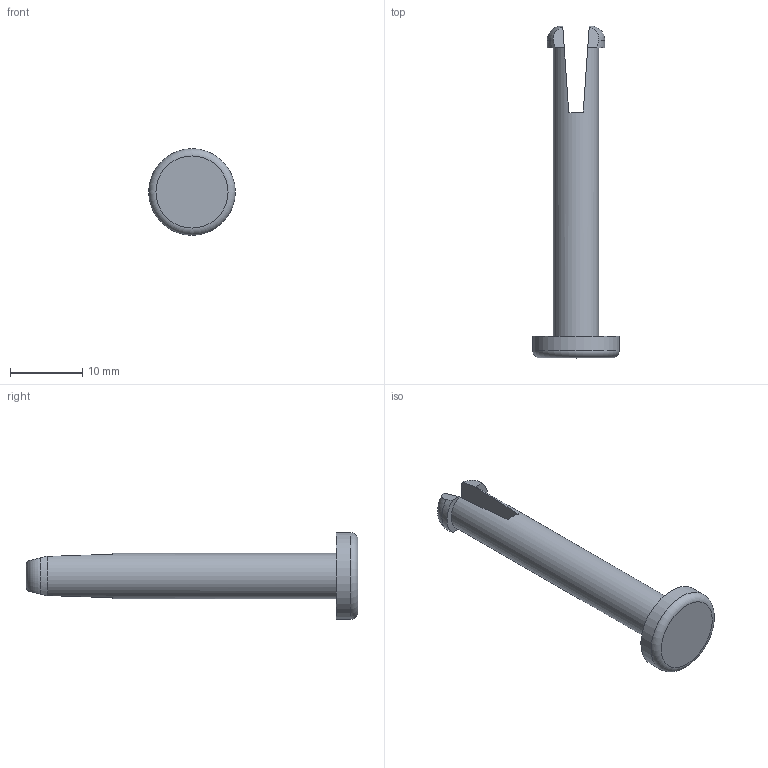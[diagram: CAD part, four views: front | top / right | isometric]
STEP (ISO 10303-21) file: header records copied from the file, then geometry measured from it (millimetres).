
FILE_DESCRIPTION(('FreeCAD Model'),'2;1');
FILE_NAME('45 Snap Pin.step','2014-08-23T00:34:39',('FreeCAD'),('FreeCAD'), 'Open CASCADE STEP processor 6.5','FreeCAD','Unknown');
FILE_SCHEMA(('AUTOMOTIVE_DESIGN_CC2 { 1 2 10303 214 -1 1 5 4 }'));
Length unit declared in the file: millimetre
Products named in the file (1): Cut002
Bounding box: 12 x 46 x 12 mm (x, y, z)
Volume: 1484.1 mm3; surface area: 1242.8 mm2
Topology: 1 solids, 1 shells, 22 faces, 56 edges, 37 vertices
Faces by surface type: plane 15, cylinder 4, torus 3
Full cylindrical faces by diameter (mm): 6.3 x1, 12 x1
Entity records: 5054 total; most frequent: CARTESIAN_POINT 4006, DIRECTION 167, ORIENTED_EDGE 112, PCURVE 112, DEFINITIONAL_REPRESENTATION 112, B_SPLINE_CURVE_WITH_KNOTS 68, EDGE_CURVE 56, SURFACE_CURVE 53
